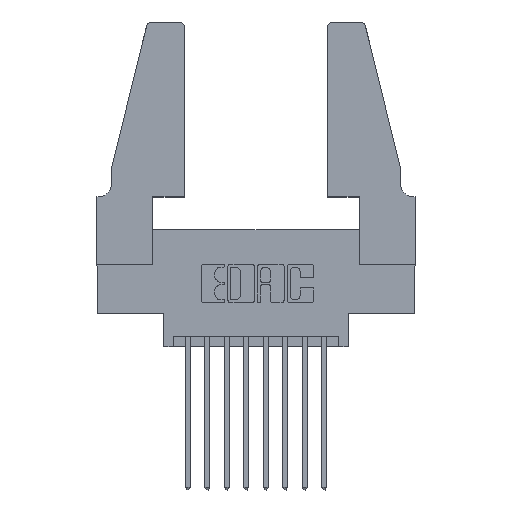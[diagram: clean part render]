
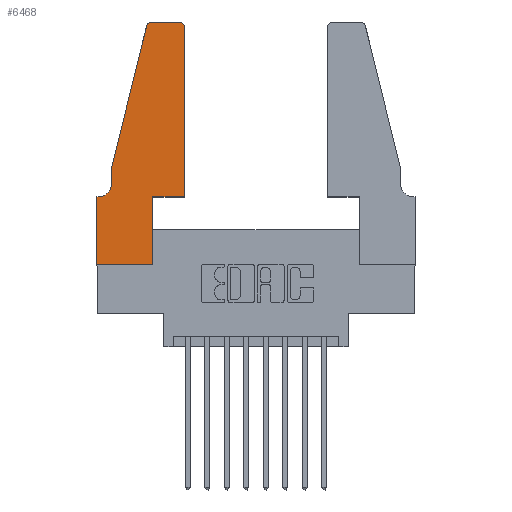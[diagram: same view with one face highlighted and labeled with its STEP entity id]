
A CAD part, top view. The second image highlights one B-rep face of the part: STEP entity #6468.
In plain terms, the highlighted planar face has unit normal (0, 0, 1).
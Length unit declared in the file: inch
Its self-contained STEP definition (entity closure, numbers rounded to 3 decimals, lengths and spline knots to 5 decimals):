
#351 = VERTEX_POINT ( 'NONE', #11398 ) ;
#369 = CIRCLE ( 'NONE', #1906, 0.03 ) ;
#460 = VECTOR ( 'NONE', #4367, 39.37008 ) ;
#597 = DIRECTION ( 'NONE',  ( 1., 0., 0. ) ) ;
#652 = LINE ( 'NONE', #2533, #3072 ) ;
#655 = ORIENTED_EDGE ( 'NONE', *, *, #8999, .T. ) ;
#676 = VECTOR ( 'NONE', #12211, 39.37008 ) ;
#718 = DIRECTION ( 'NONE',  ( -0.239, -0.971, 0. ) ) ;
#735 = CARTESIAN_POINT ( 'NONE',  ( 0.0755, 0.42, 0.37 ) ) ;
#766 = CARTESIAN_POINT ( 'NONE',  ( 0.4505, 1.22, 0.37 ) ) ;
#818 = DIRECTION ( 'NONE',  ( 0., 0., 1. ) ) ;
#873 = ORIENTED_EDGE ( 'NONE', *, *, #7750, .T. ) ;
#1056 = CARTESIAN_POINT ( 'NONE',  ( 0.0755, 0.5, 0.37 ) ) ;
#1326 = ORIENTED_EDGE ( 'NONE', *, *, #7501, .T. ) ;
#1381 = VERTEX_POINT ( 'NONE', #12332 ) ;
#1505 = CARTESIAN_POINT ( 'NONE',  ( 0., 0.35, 0.37 ) ) ;
#1781 = LINE ( 'NONE', #11868, #12594 ) ;
#1899 = EDGE_LOOP ( 'NONE', ( #3673, #12339, #5330, #3758, #655, #7213, #3902, #1326, #5823, #6192, #873, #5418 ) ) ;
#1903 = VECTOR ( 'NONE', #7048, 39.37008 ) ;
#1906 = AXIS2_PLACEMENT_3D ( 'NONE', #10300, #4242, #11271 ) ;
#1918 = LINE ( 'NONE', #7464, #12413 ) ;
#2244 = CARTESIAN_POINT ( 'NONE',  ( 0.0055, 0.42, 0.37 ) ) ;
#2533 = CARTESIAN_POINT ( 'NONE',  ( 0.0755, 0.35, 0.37 ) ) ;
#2567 = EDGE_CURVE ( 'NONE', #10456, #7651, #2997, .T. ) ;
#2997 = LINE ( 'NONE', #10002, #5485 ) ;
#3072 = VECTOR ( 'NONE', #10685, 39.37008 ) ;
#3296 = DIRECTION ( 'NONE',  ( -1., 0., 0. ) ) ;
#3369 = DIRECTION ( 'NONE',  ( 1., 0., 0. ) ) ;
#3631 = DIRECTION ( 'NONE',  ( 0., 0., 1. ) ) ;
#3673 = ORIENTED_EDGE ( 'NONE', *, *, #12055, .T. ) ;
#3758 = ORIENTED_EDGE ( 'NONE', *, *, #8892, .T. ) ;
#3902 = ORIENTED_EDGE ( 'NONE', *, *, #2567, .T. ) ;
#4135 = CIRCLE ( 'NONE', #4542, 0.03 ) ;
#4185 = CARTESIAN_POINT ( 'NONE',  ( 0.2865, 0., 0.37 ) ) ;
#4216 = LINE ( 'NONE', #8911, #11922 ) ;
#4242 = DIRECTION ( 'NONE',  ( 0., 0., 1. ) ) ;
#4367 = DIRECTION ( 'NONE',  ( 0., 1., 0. ) ) ;
#4368 = LINE ( 'NONE', #13037, #1903 ) ;
#4542 = AXIS2_PLACEMENT_3D ( 'NONE', #6993, #818, #8025 ) ;
#4750 = CARTESIAN_POINT ( 'NONE',  ( 0., 0.35, 0.37 ) ) ;
#5330 = ORIENTED_EDGE ( 'NONE', *, *, #11158, .T. ) ;
#5382 = LINE ( 'NONE', #8973, #7722 ) ;
#5418 = ORIENTED_EDGE ( 'NONE', *, *, #8931, .T. ) ;
#5485 = VECTOR ( 'NONE', #10684, 39.37008 ) ;
#5823 = ORIENTED_EDGE ( 'NONE', *, *, #11531, .T. ) ;
#5869 = DIRECTION ( 'NONE',  ( 1., 0., 0. ) ) ;
#5989 = LINE ( 'NONE', #11393, #460 ) ;
#6099 = AXIS2_PLACEMENT_3D ( 'NONE', #2244, #9455, #3296 ) ;
#6179 = VERTEX_POINT ( 'NONE', #12353 ) ;
#6192 = ORIENTED_EDGE ( 'NONE', *, *, #9920, .T. ) ;
#6468 = ADVANCED_FACE ( 'NONE', ( #11319 ), #12776, .T. ) ;
#6582 = VERTEX_POINT ( 'NONE', #766 ) ;
#6993 = CARTESIAN_POINT ( 'NONE',  ( 0.284, 1.22, 0.37 ) ) ;
#7048 = DIRECTION ( 'NONE',  ( -1., 0., 0. ) ) ;
#7213 = ORIENTED_EDGE ( 'NONE', *, *, #9819, .T. ) ;
#7326 = VERTEX_POINT ( 'NONE', #4185 ) ;
#7408 = AXIS2_PLACEMENT_3D ( 'NONE', #4750, #3631, #597 ) ;
#7464 = CARTESIAN_POINT ( 'NONE',  ( 0., 0., 0.37 ) ) ;
#7501 = EDGE_CURVE ( 'NONE', #7651, #7326, #1918, .T. ) ;
#7569 = CARTESIAN_POINT ( 'NONE',  ( 0.4205, 1.25, 0.37 ) ) ;
#7651 = VERTEX_POINT ( 'NONE', #10678 ) ;
#7722 = VECTOR ( 'NONE', #718, 39.37008 ) ;
#7750 = EDGE_CURVE ( 'NONE', #8853, #6582, #4216, .T. ) ;
#7823 = VERTEX_POINT ( 'NONE', #735 ) ;
#7933 = CIRCLE ( 'NONE', #6099, 0.07 ) ;
#8025 = DIRECTION ( 'NONE',  ( 1., 0., 0. ) ) ;
#8088 = CARTESIAN_POINT ( 'NONE',  ( 0.25487, 1.22718, 0.37 ) ) ;
#8238 = VERTEX_POINT ( 'NONE', #7569 ) ;
#8393 = EDGE_CURVE ( 'NONE', #351, #10051, #4135, .T. ) ;
#8420 = VERTEX_POINT ( 'NONE', #13026 ) ;
#8853 = VERTEX_POINT ( 'NONE', #13158 ) ;
#8892 = EDGE_CURVE ( 'NONE', #8420, #7823, #9221, .T. ) ;
#8911 = CARTESIAN_POINT ( 'NONE',  ( 0.4505, 0.35, 0.37 ) ) ;
#8931 = EDGE_CURVE ( 'NONE', #6582, #8238, #369, .T. ) ;
#8973 = CARTESIAN_POINT ( 'NONE',  ( 0.0755, 0.5, 0.37 ) ) ;
#8999 = EDGE_CURVE ( 'NONE', #7823, #6179, #7933, .T. ) ;
#9221 = LINE ( 'NONE', #1056, #676 ) ;
#9455 = DIRECTION ( 'NONE',  ( 0., 0., -1. ) ) ;
#9819 = EDGE_CURVE ( 'NONE', #6179, #10456, #652, .T. ) ;
#9920 = EDGE_CURVE ( 'NONE', #1381, #8853, #1781, .T. ) ;
#10002 = CARTESIAN_POINT ( 'NONE',  ( 0., 0., 0.37 ) ) ;
#10051 = VERTEX_POINT ( 'NONE', #8088 ) ;
#10300 = CARTESIAN_POINT ( 'NONE',  ( 0.4205, 1.22, 0.37 ) ) ;
#10456 = VERTEX_POINT ( 'NONE', #1505 ) ;
#10678 = CARTESIAN_POINT ( 'NONE',  ( 0., 0., 0.37 ) ) ;
#10684 = DIRECTION ( 'NONE',  ( 0., -1., 0. ) ) ;
#10685 = DIRECTION ( 'NONE',  ( -1., 0., 0. ) ) ;
#10853 = DIRECTION ( 'NONE',  ( 0., 1., 0. ) ) ;
#11158 = EDGE_CURVE ( 'NONE', #10051, #8420, #5382, .T. ) ;
#11271 = DIRECTION ( 'NONE',  ( 1., 0., 0. ) ) ;
#11319 = FACE_OUTER_BOUND ( 'NONE', #1899, .T. ) ;
#11393 = CARTESIAN_POINT ( 'NONE',  ( 0.2865, 0.35, 0.37 ) ) ;
#11398 = CARTESIAN_POINT ( 'NONE',  ( 0.284, 1.25, 0.37 ) ) ;
#11531 = EDGE_CURVE ( 'NONE', #7326, #1381, #5989, .T. ) ;
#11868 = CARTESIAN_POINT ( 'NONE',  ( 0.4505, 0.35, 0.37 ) ) ;
#11922 = VECTOR ( 'NONE', #10853, 39.37008 ) ;
#12055 = EDGE_CURVE ( 'NONE', #8238, #351, #4368, .T. ) ;
#12211 = DIRECTION ( 'NONE',  ( 0., -1., 0. ) ) ;
#12332 = CARTESIAN_POINT ( 'NONE',  ( 0.2865, 0.35, 0.37 ) ) ;
#12339 = ORIENTED_EDGE ( 'NONE', *, *, #8393, .T. ) ;
#12353 = CARTESIAN_POINT ( 'NONE',  ( 0.0055, 0.35, 0.37 ) ) ;
#12413 = VECTOR ( 'NONE', #3369, 39.37008 ) ;
#12594 = VECTOR ( 'NONE', #5869, 39.37008 ) ;
#12776 = PLANE ( 'NONE',  #7408 ) ;
#13026 = CARTESIAN_POINT ( 'NONE',  ( 0.0755, 0.5, 0.37 ) ) ;
#13037 = CARTESIAN_POINT ( 'NONE',  ( 0.2605, 1.25, 0.37 ) ) ;
#13158 = CARTESIAN_POINT ( 'NONE',  ( 0.4505, 0.35, 0.37 ) ) ;
